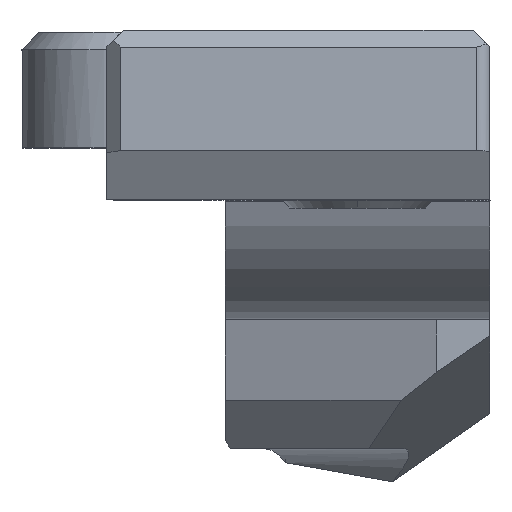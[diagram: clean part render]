
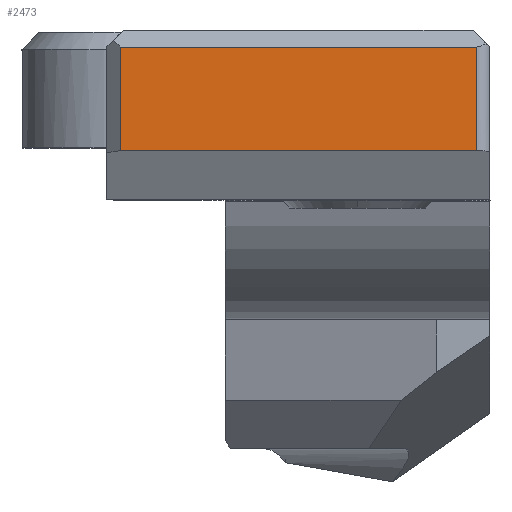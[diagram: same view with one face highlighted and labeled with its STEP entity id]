
A CAD part, left-side view. The second image highlights one B-rep face of the part: STEP entity #2473.
In plain terms, the highlighted planar face has unit normal (-1, 0, 0).
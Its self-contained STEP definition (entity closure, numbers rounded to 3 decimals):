
#8 = VECTOR ( 'NONE', #2165, 1000. ) ;
#110 = ORIENTED_EDGE ( 'NONE', *, *, #1153, .T. ) ;
#320 = DIRECTION ( 'NONE',  ( 0., 0., -1. ) ) ;
#327 = EDGE_LOOP ( 'NONE', ( #2512, #1495, #110, #2320 ) ) ;
#500 = CARTESIAN_POINT ( 'NONE',  ( -100.947, -14.561, 22.853 ) ) ;
#684 = CARTESIAN_POINT ( 'NONE',  ( -100.947, -25.061, 22.853 ) ) ;
#700 = DIRECTION ( 'NONE',  ( 0., -1., 0. ) ) ;
#848 = LINE ( 'NONE', #1288, #919 ) ;
#849 = CARTESIAN_POINT ( 'NONE',  ( -100.947, -14.561, 22.509 ) ) ;
#918 = EDGE_CURVE ( 'NONE', #2358, #1538, #2146, .T. ) ;
#919 = VECTOR ( 'NONE', #1896, 1000. ) ;
#1105 = DIRECTION ( 'NONE',  ( -1., 0., 0. ) ) ;
#1153 = EDGE_CURVE ( 'NONE', #1156, #1523, #2373, .T. ) ;
#1156 = VERTEX_POINT ( 'NONE', #500 ) ;
#1288 = CARTESIAN_POINT ( 'NONE',  ( -100.947, -24.971, 22.853 ) ) ;
#1316 = PLANE ( 'NONE',  #2327 ) ;
#1495 = ORIENTED_EDGE ( 'NONE', *, *, #2348, .T. ) ;
#1523 = VERTEX_POINT ( 'NONE', #1903 ) ;
#1538 = VERTEX_POINT ( 'NONE', #2124 ) ;
#1539 = EDGE_CURVE ( 'NONE', #1523, #1538, #2370, .T. ) ;
#1562 = CARTESIAN_POINT ( 'NONE',  ( -100.947, -25.061, 20.051 ) ) ;
#1569 = VECTOR ( 'NONE', #320, 1000. ) ;
#1803 = FACE_OUTER_BOUND ( 'NONE', #327, .T. ) ;
#1874 = VECTOR ( 'NONE', #1946, 1000. ) ;
#1896 = DIRECTION ( 'NONE',  ( 0., 1., 0. ) ) ;
#1903 = CARTESIAN_POINT ( 'NONE',  ( -100.947, -14.561, 19.803 ) ) ;
#1929 = CARTESIAN_POINT ( 'NONE',  ( -100.947, -62.008, 19.803 ) ) ;
#1946 = DIRECTION ( 'NONE',  ( 0., 0., -1. ) ) ;
#2124 = CARTESIAN_POINT ( 'NONE',  ( -100.947, -25.061, 19.803 ) ) ;
#2146 = LINE ( 'NONE', #1562, #1569 ) ;
#2165 = DIRECTION ( 'NONE',  ( 0., -1., 0. ) ) ;
#2320 = ORIENTED_EDGE ( 'NONE', *, *, #1539, .T. ) ;
#2327 = AXIS2_PLACEMENT_3D ( 'NONE', #2577, #1105, #700 ) ;
#2348 = EDGE_CURVE ( 'NONE', #2358, #1156, #848, .T. ) ;
#2358 = VERTEX_POINT ( 'NONE', #684 ) ;
#2370 = LINE ( 'NONE', #1929, #8 ) ;
#2373 = LINE ( 'NONE', #849, #1874 ) ;
#2473 = ADVANCED_FACE ( 'NONE', ( #1803 ), #1316, .T. ) ;
#2512 = ORIENTED_EDGE ( 'NONE', *, *, #918, .F. ) ;
#2577 = CARTESIAN_POINT ( 'NONE',  ( -100.947, -24.971, 22.509 ) ) ;
